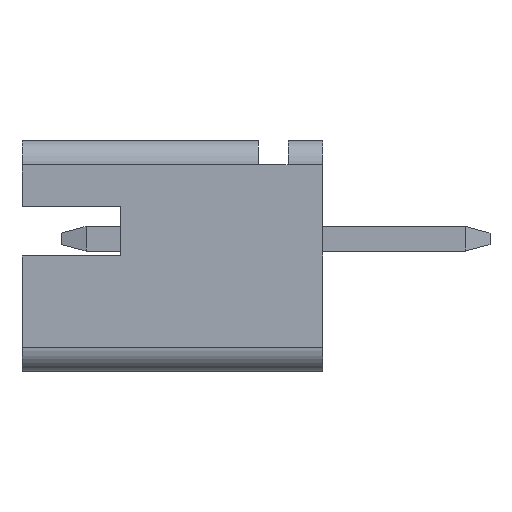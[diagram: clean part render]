
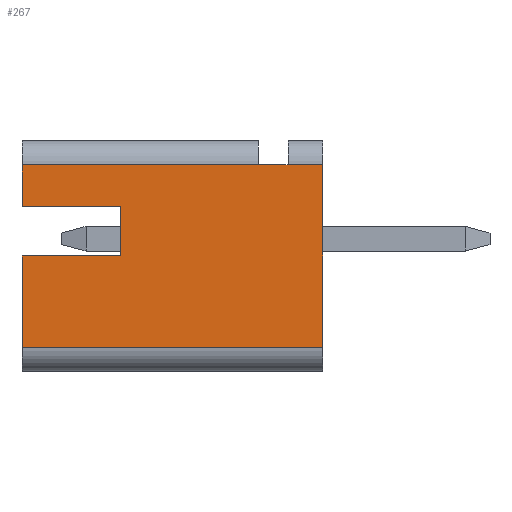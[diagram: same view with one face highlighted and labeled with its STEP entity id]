
A CAD part, left-side view. The second image highlights one B-rep face of the part: STEP entity #267.
In plain terms, the highlighted planar face has unit normal (-1, 0, 0).
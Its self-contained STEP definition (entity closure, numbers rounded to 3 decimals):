
#28 = DIRECTION ( 'NONE',  ( 0., 0., -1. ) ) ;
#67 = LINE ( 'NONE', #3137, #1801 ) ;
#97 = ORIENTED_EDGE ( 'NONE', *, *, #1551, .F. ) ;
#135 = VERTEX_POINT ( 'NONE', #3337 ) ;
#209 = LINE ( 'NONE', #3636, #1554 ) ;
#213 = ORIENTED_EDGE ( 'NONE', *, *, #2989, .F. ) ;
#218 = EDGE_CURVE ( 'NONE', #135, #2945, #842, .T. ) ;
#267 = ADVANCED_FACE ( 'NONE', ( #1238 ), #657, .F. ) ;
#466 = VERTEX_POINT ( 'NONE', #1719 ) ;
#472 = CARTESIAN_POINT ( 'NONE',  ( -2., 1.3, 1.5 ) ) ;
#485 = VECTOR ( 'NONE', #2159, 1000. ) ;
#545 = DIRECTION ( 'NONE',  ( 0., -1., 0. ) ) ;
#657 = PLANE ( 'NONE',  #743 ) ;
#743 = AXIS2_PLACEMENT_3D ( 'NONE', #3102, #2180, #28 ) ;
#768 = LINE ( 'NONE', #1447, #3411 ) ;
#842 = LINE ( 'NONE', #906, #485 ) ;
#848 = LINE ( 'NONE', #2165, #3579 ) ;
#856 = EDGE_CURVE ( 'NONE', #2284, #1360, #1309, .T. ) ;
#906 = CARTESIAN_POINT ( 'NONE',  ( -2., 0., 1.5 ) ) ;
#923 = VECTOR ( 'NONE', #1166, 1000. ) ;
#1008 = CARTESIAN_POINT ( 'NONE',  ( -2., 4.1, 0.65 ) ) ;
#1027 = DIRECTION ( 'NONE',  ( 0., 0., 1. ) ) ;
#1068 = EDGE_CURVE ( 'NONE', #1697, #1816, #3210, .T. ) ;
#1092 = EDGE_LOOP ( 'NONE', ( #213, #1401, #1931, #3949, #97, #2866, #1582, #1098, #1826, #2591 ) ) ;
#1098 = ORIENTED_EDGE ( 'NONE', *, *, #3952, .F. ) ;
#1166 = DIRECTION ( 'NONE',  ( 0., -1., 0. ) ) ;
#1238 = FACE_OUTER_BOUND ( 'NONE', #1092, .T. ) ;
#1309 = LINE ( 'NONE', #1008, #4006 ) ;
#1346 = VERTEX_POINT ( 'NONE', #472 ) ;
#1360 = VERTEX_POINT ( 'NONE', #2373 ) ;
#1401 = ORIENTED_EDGE ( 'NONE', *, *, #3686, .T. ) ;
#1447 = CARTESIAN_POINT ( 'NONE',  ( -2., 6.1, 0.65 ) ) ;
#1452 = DIRECTION ( 'NONE',  ( 0., 0., -1. ) ) ;
#1485 = VECTOR ( 'NONE', #3962, 1000. ) ;
#1551 = EDGE_CURVE ( 'NONE', #1346, #2945, #2188, .T. ) ;
#1554 = VECTOR ( 'NONE', #1452, 1000. ) ;
#1582 = ORIENTED_EDGE ( 'NONE', *, *, #1068, .F. ) ;
#1697 = VERTEX_POINT ( 'NONE', #2306 ) ;
#1719 = CARTESIAN_POINT ( 'NONE',  ( -2., 6.1, -2.2 ) ) ;
#1801 = VECTOR ( 'NONE', #2811, 1000. ) ;
#1816 = VERTEX_POINT ( 'NONE', #3717 ) ;
#1826 = ORIENTED_EDGE ( 'NONE', *, *, #856, .F. ) ;
#1931 = ORIENTED_EDGE ( 'NONE', *, *, #3538, .F. ) ;
#1983 = CARTESIAN_POINT ( 'NONE',  ( -2., 6.1, 2. ) ) ;
#2096 = LINE ( 'NONE', #3064, #1485 ) ;
#2118 = VERTEX_POINT ( 'NONE', #3438 ) ;
#2159 = DIRECTION ( 'NONE',  ( 0., 1., 0. ) ) ;
#2165 = CARTESIAN_POINT ( 'NONE',  ( -2., 0., -2.2 ) ) ;
#2180 = DIRECTION ( 'NONE',  ( 1., 0., 0. ) ) ;
#2188 = LINE ( 'NONE', #3432, #923 ) ;
#2245 = EDGE_CURVE ( 'NONE', #2118, #2284, #67, .T. ) ;
#2284 = VERTEX_POINT ( 'NONE', #2968 ) ;
#2306 = CARTESIAN_POINT ( 'NONE',  ( -2., 6.1, 0.65 ) ) ;
#2373 = CARTESIAN_POINT ( 'NONE',  ( -2., 4.1, 0.65 ) ) ;
#2551 = DIRECTION ( 'NONE',  ( 0., 1., 0. ) ) ;
#2591 = ORIENTED_EDGE ( 'NONE', *, *, #2245, .F. ) ;
#2665 = VECTOR ( 'NONE', #2551, 1000. ) ;
#2675 = DIRECTION ( 'NONE',  ( 0., 1., 0. ) ) ;
#2811 = DIRECTION ( 'NONE',  ( 0., -1., 0. ) ) ;
#2866 = ORIENTED_EDGE ( 'NONE', *, *, #3344, .T. ) ;
#2914 = VERTEX_POINT ( 'NONE', #3535 ) ;
#2945 = VERTEX_POINT ( 'NONE', #3672 ) ;
#2968 = CARTESIAN_POINT ( 'NONE',  ( -2., 4.1, -0.35 ) ) ;
#2989 = EDGE_CURVE ( 'NONE', #466, #2118, #2096, .T. ) ;
#3064 = CARTESIAN_POINT ( 'NONE',  ( -2., 6.1, -0.35 ) ) ;
#3102 = CARTESIAN_POINT ( 'NONE',  ( -2., 0., 0. ) ) ;
#3137 = CARTESIAN_POINT ( 'NONE',  ( -2., 6.1, -0.35 ) ) ;
#3210 = LINE ( 'NONE', #1983, #3255 ) ;
#3255 = VECTOR ( 'NONE', #1027, 1000. ) ;
#3337 = CARTESIAN_POINT ( 'NONE',  ( -2., 0., 1.5 ) ) ;
#3344 = EDGE_CURVE ( 'NONE', #1346, #1816, #3471, .T. ) ;
#3411 = VECTOR ( 'NONE', #2675, 1000. ) ;
#3432 = CARTESIAN_POINT ( 'NONE',  ( -2., 1.3, 1.5 ) ) ;
#3438 = CARTESIAN_POINT ( 'NONE',  ( -2., 6.1, -0.35 ) ) ;
#3471 = LINE ( 'NONE', #3536, #2665 ) ;
#3535 = CARTESIAN_POINT ( 'NONE',  ( -2., 0., -2.2 ) ) ;
#3536 = CARTESIAN_POINT ( 'NONE',  ( -2., 0., 1.5 ) ) ;
#3538 = EDGE_CURVE ( 'NONE', #135, #2914, #209, .T. ) ;
#3579 = VECTOR ( 'NONE', #545, 1000. ) ;
#3636 = CARTESIAN_POINT ( 'NONE',  ( -2., 0., 2. ) ) ;
#3672 = CARTESIAN_POINT ( 'NONE',  ( -2., 0.7, 1.5 ) ) ;
#3686 = EDGE_CURVE ( 'NONE', #466, #2914, #848, .T. ) ;
#3717 = CARTESIAN_POINT ( 'NONE',  ( -2., 6.1, 1.5 ) ) ;
#3870 = DIRECTION ( 'NONE',  ( 0., 0., 1. ) ) ;
#3949 = ORIENTED_EDGE ( 'NONE', *, *, #218, .T. ) ;
#3952 = EDGE_CURVE ( 'NONE', #1360, #1697, #768, .T. ) ;
#3962 = DIRECTION ( 'NONE',  ( 0., 0., 1. ) ) ;
#4006 = VECTOR ( 'NONE', #3870, 1000. ) ;
